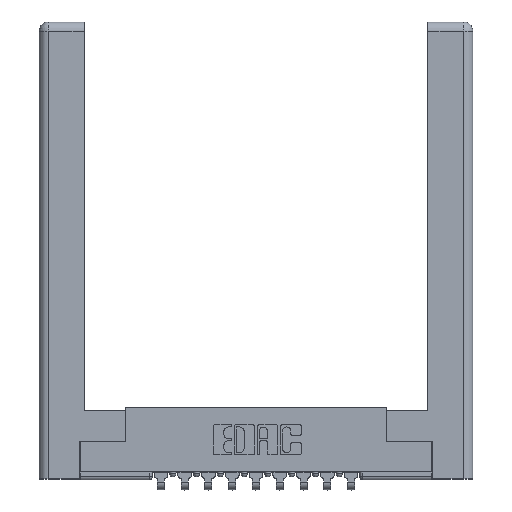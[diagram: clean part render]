
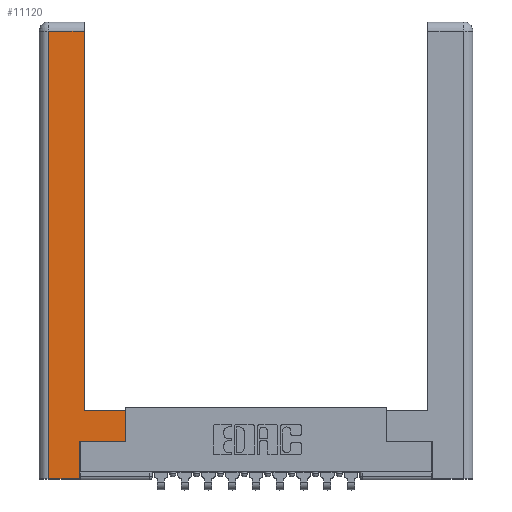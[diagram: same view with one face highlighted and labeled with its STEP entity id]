
A CAD part, top view. The second image highlights one B-rep face of the part: STEP entity #11120.
In plain terms, the highlighted planar face has unit normal (0, 0, 1).
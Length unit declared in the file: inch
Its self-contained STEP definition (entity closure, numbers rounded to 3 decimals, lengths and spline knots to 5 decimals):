
#116 = VERTEX_POINT ( 'NONE', #10855 ) ;
#170 = CARTESIAN_POINT ( 'NONE',  ( 0.0615, 2.94, 0. ) ) ;
#277 = VECTOR ( 'NONE', #13670, 39.37008 ) ;
#649 = DIRECTION ( 'NONE',  ( 0., -1., 0. ) ) ;
#669 = ORIENTED_EDGE ( 'NONE', *, *, #12670, .T. ) ;
#984 = CARTESIAN_POINT ( 'NONE',  ( 0.295, 0.45, 0. ) ) ;
#1359 = VECTOR ( 'NONE', #11035, 39.37008 ) ;
#1718 = VERTEX_POINT ( 'NONE', #10638 ) ;
#2029 = AXIS2_PLACEMENT_3D ( 'NONE', #8700, #3098, #6441 ) ;
#2048 = VERTEX_POINT ( 'NONE', #14414 ) ;
#2850 = CARTESIAN_POINT ( 'NONE',  ( 0.0615, 0., 0. ) ) ;
#2902 = LINE ( 'NONE', #984, #10786 ) ;
#3098 = DIRECTION ( 'NONE',  ( 0., 0., -1. ) ) ;
#3887 = EDGE_CURVE ( 'NONE', #12680, #2048, #5308, .T. ) ;
#5308 = LINE ( 'NONE', #7062, #277 ) ;
#6216 = VERTEX_POINT ( 'NONE', #11797 ) ;
#6441 = DIRECTION ( 'NONE',  ( -1., 0., 0. ) ) ;
#6683 = ORIENTED_EDGE ( 'NONE', *, *, #10604, .T. ) ;
#6822 = EDGE_LOOP ( 'NONE', ( #9128, #9329, #14158, #6683, #9698, #12864, #11311, #669 ) ) ;
#7062 = CARTESIAN_POINT ( 'NONE',  ( 0.565, 0.245, 0. ) ) ;
#7487 = CARTESIAN_POINT ( 'NONE',  ( 0.0615, 2.94, 0. ) ) ;
#7726 = EDGE_CURVE ( 'NONE', #10004, #11272, #12192, .T. ) ;
#7980 = CARTESIAN_POINT ( 'NONE',  ( 0.565, 0.45, 0. ) ) ;
#8067 = LINE ( 'NONE', #7980, #14535 ) ;
#8100 = CARTESIAN_POINT ( 'NONE',  ( 0.295, 0.45, 0. ) ) ;
#8102 = EDGE_CURVE ( 'NONE', #6216, #12680, #14197, .T. ) ;
#8369 = DIRECTION ( 'NONE',  ( 1., 0., 0. ) ) ;
#8570 = VECTOR ( 'NONE', #11964, 39.37008 ) ;
#8695 = CARTESIAN_POINT ( 'NONE',  ( 0.265, 0.245, 0. ) ) ;
#8700 = CARTESIAN_POINT ( 'NONE',  ( 0., 0., 0. ) ) ;
#8874 = EDGE_CURVE ( 'NONE', #11272, #116, #12925, .T. ) ;
#9068 = VECTOR ( 'NONE', #9542, 39.37008 ) ;
#9128 = ORIENTED_EDGE ( 'NONE', *, *, #11387, .T. ) ;
#9172 = DIRECTION ( 'NONE',  ( 0., 1., 0. ) ) ;
#9329 = ORIENTED_EDGE ( 'NONE', *, *, #7726, .T. ) ;
#9542 = DIRECTION ( 'NONE',  ( 0., 1., 0. ) ) ;
#9627 = LINE ( 'NONE', #13945, #14230 ) ;
#9698 = ORIENTED_EDGE ( 'NONE', *, *, #8102, .T. ) ;
#9969 = VERTEX_POINT ( 'NONE', #8100 ) ;
#10004 = VERTEX_POINT ( 'NONE', #11420 ) ;
#10604 = EDGE_CURVE ( 'NONE', #116, #6216, #9627, .T. ) ;
#10638 = CARTESIAN_POINT ( 'NONE',  ( 0.565, 0.45, 0. ) ) ;
#10786 = VECTOR ( 'NONE', #12026, 39.37008 ) ;
#10851 = PLANE ( 'NONE',  #2029 ) ;
#10855 = CARTESIAN_POINT ( 'NONE',  ( 0.0615, 0., 0. ) ) ;
#10961 = CARTESIAN_POINT ( 'NONE',  ( 0.295, 3., 0. ) ) ;
#11035 = DIRECTION ( 'NONE',  ( 0., 1., 0. ) ) ;
#11120 = ADVANCED_FACE ( 'NONE', ( #14425 ), #10851, .F. ) ;
#11272 = VERTEX_POINT ( 'NONE', #170 ) ;
#11311 = ORIENTED_EDGE ( 'NONE', *, *, #12823, .T. ) ;
#11387 = EDGE_CURVE ( 'NONE', #9969, #10004, #14319, .T. ) ;
#11420 = CARTESIAN_POINT ( 'NONE',  ( 0.295, 2.94, 0. ) ) ;
#11797 = CARTESIAN_POINT ( 'NONE',  ( 0.265, 0., 0. ) ) ;
#11964 = DIRECTION ( 'NONE',  ( -1., 0., 0. ) ) ;
#12026 = DIRECTION ( 'NONE',  ( -1., 0., 0. ) ) ;
#12176 = CARTESIAN_POINT ( 'NONE',  ( 0.265, 0.245, 0. ) ) ;
#12192 = LINE ( 'NONE', #7487, #8570 ) ;
#12583 = VECTOR ( 'NONE', #649, 39.37008 ) ;
#12670 = EDGE_CURVE ( 'NONE', #1718, #9969, #2902, .T. ) ;
#12680 = VERTEX_POINT ( 'NONE', #12176 ) ;
#12823 = EDGE_CURVE ( 'NONE', #2048, #1718, #8067, .T. ) ;
#12864 = ORIENTED_EDGE ( 'NONE', *, *, #3887, .T. ) ;
#12925 = LINE ( 'NONE', #2850, #12583 ) ;
#13670 = DIRECTION ( 'NONE',  ( 1., 0., 0. ) ) ;
#13945 = CARTESIAN_POINT ( 'NONE',  ( 0.265, 0., 0. ) ) ;
#14158 = ORIENTED_EDGE ( 'NONE', *, *, #8874, .T. ) ;
#14197 = LINE ( 'NONE', #8695, #9068 ) ;
#14230 = VECTOR ( 'NONE', #8369, 39.37008 ) ;
#14319 = LINE ( 'NONE', #10961, #1359 ) ;
#14414 = CARTESIAN_POINT ( 'NONE',  ( 0.565, 0.245, 0. ) ) ;
#14425 = FACE_OUTER_BOUND ( 'NONE', #6822, .T. ) ;
#14535 = VECTOR ( 'NONE', #9172, 39.37008 ) ;
